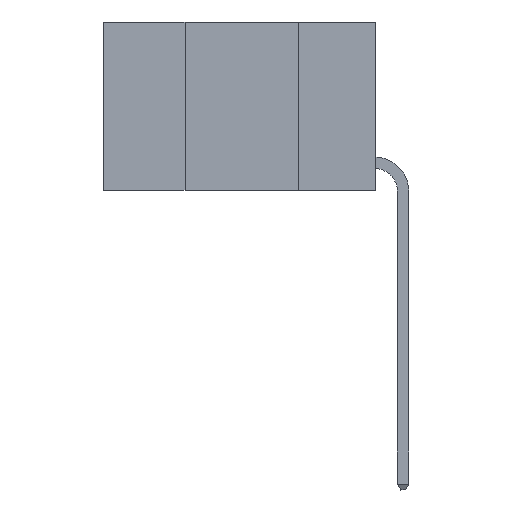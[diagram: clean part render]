
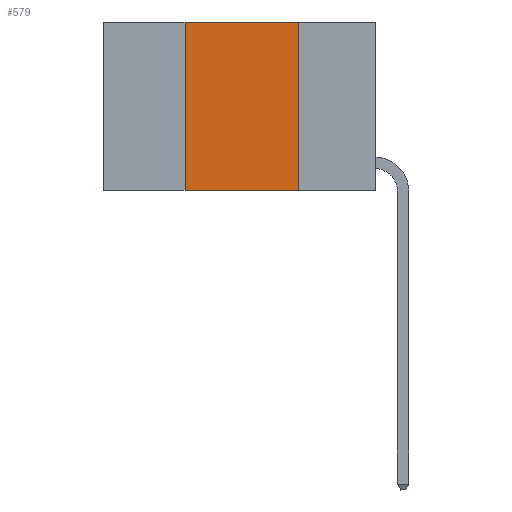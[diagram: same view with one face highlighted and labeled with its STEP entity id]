
A CAD part, left-side view. The second image highlights one B-rep face of the part: STEP entity #579.
In plain terms, the highlighted planar face has unit normal (-1, 0, 0).
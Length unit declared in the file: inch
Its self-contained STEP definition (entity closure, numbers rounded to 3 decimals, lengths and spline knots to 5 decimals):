
#103 = CARTESIAN_POINT ( 'NONE',  ( 0., 0.17, 0. ) ) ;
#186 = CARTESIAN_POINT ( 'NONE',  ( 0., 0.6, 0. ) ) ;
#579 = ADVANCED_FACE ( 'NONE', ( #6732 ), #11304, .F. ) ;
#853 = DIRECTION ( 'NONE',  ( 1., 0., 0. ) ) ;
#953 = LINE ( 'NONE', #8138, #4791 ) ;
#1279 = VECTOR ( 'NONE', #13261, 39.37008 ) ;
#1348 = VERTEX_POINT ( 'NONE', #14215 ) ;
#1509 = ORIENTED_EDGE ( 'NONE', *, *, #7377, .F. ) ;
#1788 = ORIENTED_EDGE ( 'NONE', *, *, #2476, .T. ) ;
#2476 = EDGE_CURVE ( 'NONE', #14833, #3783, #7740, .T. ) ;
#2713 = LINE ( 'NONE', #186, #3564 ) ;
#2781 = DIRECTION ( 'NONE',  ( 0., -1., 0. ) ) ;
#2816 = VERTEX_POINT ( 'NONE', #13689 ) ;
#3123 = VECTOR ( 'NONE', #11009, 39.37008 ) ;
#3564 = VECTOR ( 'NONE', #2781, 39.37008 ) ;
#3783 = VERTEX_POINT ( 'NONE', #6139 ) ;
#3924 = CARTESIAN_POINT ( 'NONE',  ( 0., 0.6, 0. ) ) ;
#4791 = VECTOR ( 'NONE', #6974, 39.37008 ) ;
#5078 = LINE ( 'NONE', #103, #1279 ) ;
#6139 = CARTESIAN_POINT ( 'NONE',  ( 0., 0.17, -0.37 ) ) ;
#6168 = ORIENTED_EDGE ( 'NONE', *, *, #12800, .F. ) ;
#6513 = AXIS2_PLACEMENT_3D ( 'NONE', #3924, #853, #6813 ) ;
#6571 = EDGE_LOOP ( 'NONE', ( #1509, #6168, #14091, #1788 ) ) ;
#6590 = CARTESIAN_POINT ( 'NONE',  ( 0., 0.6, -0.37 ) ) ;
#6732 = FACE_OUTER_BOUND ( 'NONE', #6571, .T. ) ;
#6813 = DIRECTION ( 'NONE',  ( 0., 0., -1. ) ) ;
#6974 = DIRECTION ( 'NONE',  ( 0., 0., 1. ) ) ;
#7377 = EDGE_CURVE ( 'NONE', #1348, #3783, #5078, .T. ) ;
#7740 = LINE ( 'NONE', #6590, #3123 ) ;
#8138 = CARTESIAN_POINT ( 'NONE',  ( 0., 0.42, 0. ) ) ;
#10767 = CARTESIAN_POINT ( 'NONE',  ( 0., 0.42, -0.37 ) ) ;
#11009 = DIRECTION ( 'NONE',  ( 0., -1., 0. ) ) ;
#11304 = PLANE ( 'NONE',  #6513 ) ;
#12800 = EDGE_CURVE ( 'NONE', #2816, #1348, #2713, .T. ) ;
#13043 = EDGE_CURVE ( 'NONE', #14833, #2816, #953, .T. ) ;
#13261 = DIRECTION ( 'NONE',  ( 0., 0., -1. ) ) ;
#13689 = CARTESIAN_POINT ( 'NONE',  ( 0., 0.42, 0. ) ) ;
#14091 = ORIENTED_EDGE ( 'NONE', *, *, #13043, .F. ) ;
#14215 = CARTESIAN_POINT ( 'NONE',  ( 0., 0.17, 0. ) ) ;
#14833 = VERTEX_POINT ( 'NONE', #10767 ) ;
